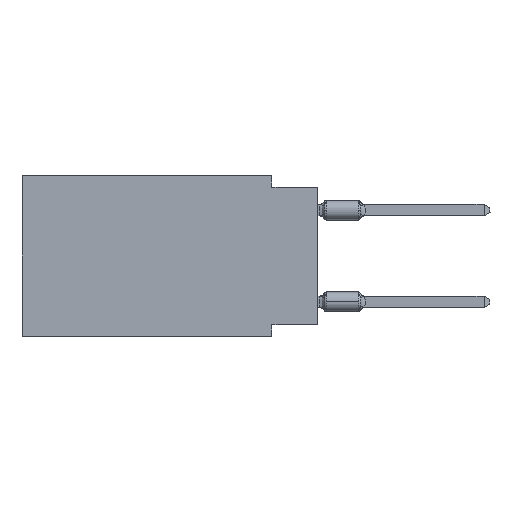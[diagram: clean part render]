
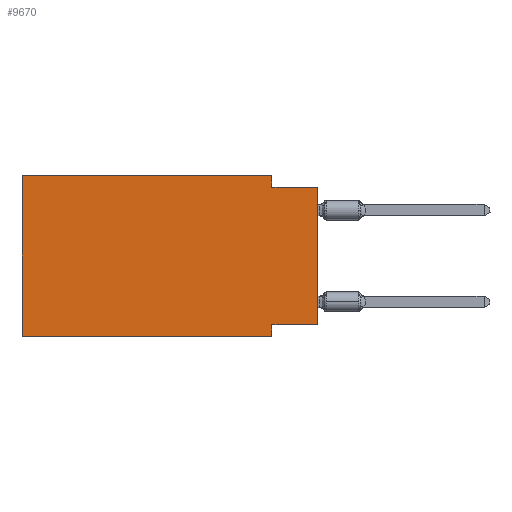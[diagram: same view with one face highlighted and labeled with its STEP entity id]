
A CAD part, left-side view. The second image highlights one B-rep face of the part: STEP entity #9670.
In plain terms, the highlighted planar face has unit normal (-1, 0, 0).
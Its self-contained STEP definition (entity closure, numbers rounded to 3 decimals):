
#290 = ORIENTED_EDGE ( 'NONE', *, *, #439, .F. ) ;
#405 = LINE ( 'NONE', #27249, #13618 ) ;
#439 = EDGE_CURVE ( 'NONE', #58146, #14633, #16628, .T. ) ;
#800 = CARTESIAN_POINT ( 'NONE',  ( 0., 2.54, -0.635 ) ) ;
#3088 = CARTESIAN_POINT ( 'NONE',  ( 0., 2.54, -8.255 ) ) ;
#6897 = ORIENTED_EDGE ( 'NONE', *, *, #40254, .F. ) ;
#7199 = FACE_OUTER_BOUND ( 'NONE', #23242, .T. ) ;
#8672 = DIRECTION ( 'NONE',  ( 0., 0., -1. ) ) ;
#9670 = ADVANCED_FACE ( 'NONE', ( #7199 ), #16064, .F. ) ;
#10061 = VECTOR ( 'NONE', #24276, 1000. ) ;
#10108 = LINE ( 'NONE', #23673, #26345 ) ;
#12172 = VECTOR ( 'NONE', #20704, 1000. ) ;
#12488 = EDGE_CURVE ( 'NONE', #45973, #45288, #55524, .T. ) ;
#13205 = CARTESIAN_POINT ( 'NONE',  ( 0., 2.54, -8.89 ) ) ;
#13618 = VECTOR ( 'NONE', #8672, 1000. ) ;
#13798 = VERTEX_POINT ( 'NONE', #18914 ) ;
#14071 = LINE ( 'NONE', #13205, #34466 ) ;
#14176 = CARTESIAN_POINT ( 'NONE',  ( 0., 0., -8.255 ) ) ;
#14536 = DIRECTION ( 'NONE',  ( 0., 0., 1. ) ) ;
#14633 = VERTEX_POINT ( 'NONE', #44029 ) ;
#15064 = LINE ( 'NONE', #51340, #28213 ) ;
#15785 = EDGE_CURVE ( 'NONE', #14633, #40317, #405, .T. ) ;
#16064 = PLANE ( 'NONE',  #47380 ) ;
#16628 = LINE ( 'NONE', #16910, #52351 ) ;
#16910 = CARTESIAN_POINT ( 'NONE',  ( 0., 16.383, 0. ) ) ;
#17334 = DIRECTION ( 'NONE',  ( 0., 0., -1. ) ) ;
#18326 = CARTESIAN_POINT ( 'NONE',  ( 0., 0., -8.255 ) ) ;
#18914 = CARTESIAN_POINT ( 'NONE',  ( 0., 0., -0.635 ) ) ;
#20704 = DIRECTION ( 'NONE',  ( 0., -1., 0. ) ) ;
#21854 = CARTESIAN_POINT ( 'NONE',  ( 0., 2.54, -8.89 ) ) ;
#23242 = EDGE_LOOP ( 'NONE', ( #50857, #50622, #40728, #290, #31933, #53484, #6897, #55287 ) ) ;
#23673 = CARTESIAN_POINT ( 'NONE',  ( 0., 16.383, 0. ) ) ;
#24276 = DIRECTION ( 'NONE',  ( 0., 0., 1. ) ) ;
#26345 = VECTOR ( 'NONE', #14536, 1000. ) ;
#27249 = CARTESIAN_POINT ( 'NONE',  ( 0., 2.54, 0. ) ) ;
#28112 = LINE ( 'NONE', #46104, #10061 ) ;
#28213 = VECTOR ( 'NONE', #38334, 1000. ) ;
#28766 = EDGE_CURVE ( 'NONE', #45973, #13798, #28112, .T. ) ;
#29565 = CARTESIAN_POINT ( 'NONE',  ( 0., 16.383, -8.89 ) ) ;
#31933 = ORIENTED_EDGE ( 'NONE', *, *, #33523, .F. ) ;
#33472 = CARTESIAN_POINT ( 'NONE',  ( 0., 16.383, 0. ) ) ;
#33523 = EDGE_CURVE ( 'NONE', #48046, #58146, #10108, .T. ) ;
#34466 = VECTOR ( 'NONE', #17334, 1000. ) ;
#34614 = DIRECTION ( 'NONE',  ( 0., -1., 0. ) ) ;
#34617 = DIRECTION ( 'NONE',  ( 1., 0., 0. ) ) ;
#38334 = DIRECTION ( 'NONE',  ( 0., -1., 0. ) ) ;
#40254 = EDGE_CURVE ( 'NONE', #45288, #46934, #14071, .T. ) ;
#40317 = VERTEX_POINT ( 'NONE', #800 ) ;
#40728 = ORIENTED_EDGE ( 'NONE', *, *, #15785, .F. ) ;
#44029 = CARTESIAN_POINT ( 'NONE',  ( 0., 2.54, 0. ) ) ;
#44793 = VECTOR ( 'NONE', #46344, 1000. ) ;
#45288 = VERTEX_POINT ( 'NONE', #3088 ) ;
#45973 = VERTEX_POINT ( 'NONE', #14176 ) ;
#46104 = CARTESIAN_POINT ( 'NONE',  ( 0., 0., 0. ) ) ;
#46344 = DIRECTION ( 'NONE',  ( 0., 1., 0. ) ) ;
#46934 = VERTEX_POINT ( 'NONE', #21854 ) ;
#47380 = AXIS2_PLACEMENT_3D ( 'NONE', #53201, #34617, #52626 ) ;
#47845 = LINE ( 'NONE', #29565, #12172 ) ;
#47972 = CARTESIAN_POINT ( 'NONE',  ( 0., 16.383, -8.89 ) ) ;
#48046 = VERTEX_POINT ( 'NONE', #47972 ) ;
#49770 = EDGE_CURVE ( 'NONE', #40317, #13798, #15064, .T. ) ;
#50588 = EDGE_CURVE ( 'NONE', #48046, #46934, #47845, .T. ) ;
#50622 = ORIENTED_EDGE ( 'NONE', *, *, #49770, .F. ) ;
#50857 = ORIENTED_EDGE ( 'NONE', *, *, #28766, .T. ) ;
#51340 = CARTESIAN_POINT ( 'NONE',  ( 0., 0., -0.635 ) ) ;
#52351 = VECTOR ( 'NONE', #34614, 1000. ) ;
#52626 = DIRECTION ( 'NONE',  ( 0., 0., -1. ) ) ;
#53201 = CARTESIAN_POINT ( 'NONE',  ( 0., 16.383, 0. ) ) ;
#53484 = ORIENTED_EDGE ( 'NONE', *, *, #50588, .T. ) ;
#55287 = ORIENTED_EDGE ( 'NONE', *, *, #12488, .F. ) ;
#55524 = LINE ( 'NONE', #18326, #44793 ) ;
#58146 = VERTEX_POINT ( 'NONE', #33472 ) ;
